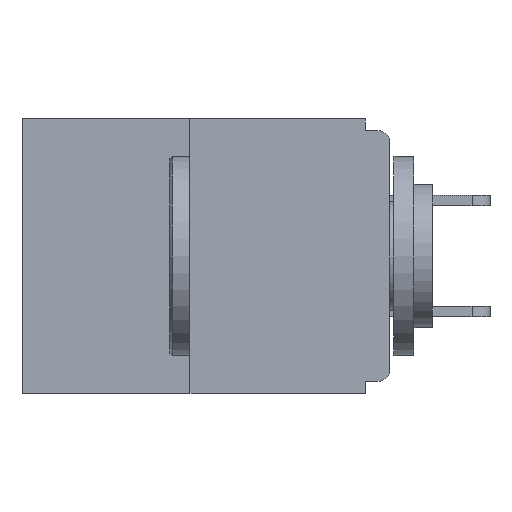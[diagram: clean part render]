
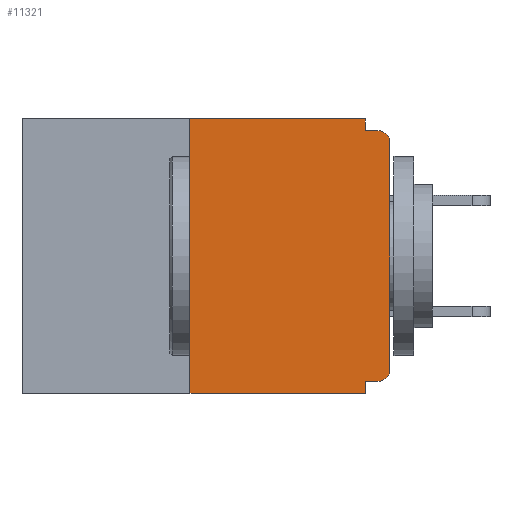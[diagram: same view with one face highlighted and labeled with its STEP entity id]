
A CAD part, left-side view. The second image highlights one B-rep face of the part: STEP entity #11321.
In plain terms, the highlighted planar face has unit normal (-1, 0, 0).
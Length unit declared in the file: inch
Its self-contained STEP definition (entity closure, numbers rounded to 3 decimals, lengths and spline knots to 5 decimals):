
#29 = DIRECTION ( 'NONE',  ( 1., 0., 0. ) ) ;
#92 = ORIENTED_EDGE ( 'NONE', *, *, #10430, .T. ) ;
#183 = DIRECTION ( 'NONE',  ( 0., 0., 1. ) ) ;
#294 = VERTEX_POINT ( 'NONE', #725 ) ;
#322 = AXIS2_PLACEMENT_3D ( 'NONE', #8437, #29, #8580 ) ;
#725 = CARTESIAN_POINT ( 'NONE',  ( 0., 0., -0.313 ) ) ;
#893 = CARTESIAN_POINT ( 'NONE',  ( 0., 0.031, -0.343 ) ) ;
#1575 = CARTESIAN_POINT ( 'NONE',  ( 0., 0.25, 0. ) ) ;
#1638 = DIRECTION ( 'NONE',  ( 0., 0., -1. ) ) ;
#2062 = ORIENTED_EDGE ( 'NONE', *, *, #11120, .T. ) ;
#2127 = LINE ( 'NONE', #3021, #7618 ) ;
#2630 = DIRECTION ( 'NONE',  ( 0., 0., -1. ) ) ;
#3021 = CARTESIAN_POINT ( 'NONE',  ( 0., 0.46, -0.343 ) ) ;
#3140 = CARTESIAN_POINT ( 'NONE',  ( 0., 0.031, -0.015 ) ) ;
#3347 = ORIENTED_EDGE ( 'NONE', *, *, #10351, .T. ) ;
#3365 = ORIENTED_EDGE ( 'NONE', *, *, #12907, .F. ) ;
#3412 = LINE ( 'NONE', #9263, #6564 ) ;
#3516 = CARTESIAN_POINT ( 'NONE',  ( 0., 0.015, -0.03 ) ) ;
#3700 = EDGE_CURVE ( 'NONE', #9054, #10824, #12797, .T. ) ;
#4074 = DIRECTION ( 'NONE',  ( 0., -1., 0. ) ) ;
#4502 = VECTOR ( 'NONE', #12166, 39.37008 ) ;
#4581 = CARTESIAN_POINT ( 'NONE',  ( 0., 0.25, 0. ) ) ;
#4733 = VECTOR ( 'NONE', #7229, 39.37008 ) ;
#4738 = DIRECTION ( 'NONE',  ( -1., 0., 0. ) ) ;
#4874 = EDGE_CURVE ( 'NONE', #5686, #12317, #10816, .T. ) ;
#5145 = CARTESIAN_POINT ( 'NONE',  ( 0., 0.46, 0. ) ) ;
#5292 = CARTESIAN_POINT ( 'NONE',  ( 0., 0.015, -0.328 ) ) ;
#5483 = VECTOR ( 'NONE', #4074, 39.37008 ) ;
#5686 = VERTEX_POINT ( 'NONE', #3140 ) ;
#5849 = ORIENTED_EDGE ( 'NONE', *, *, #12723, .F. ) ;
#5891 = DIRECTION ( 'NONE',  ( 0., 0., 1. ) ) ;
#6254 = LINE ( 'NONE', #4581, #9933 ) ;
#6564 = VECTOR ( 'NONE', #12389, 39.37008 ) ;
#7229 = DIRECTION ( 'NONE',  ( 0., -1., 0. ) ) ;
#7510 = VERTEX_POINT ( 'NONE', #8143 ) ;
#7606 = CIRCLE ( 'NONE', #13132, 0.015 ) ;
#7618 = VECTOR ( 'NONE', #11490, 39.37008 ) ;
#7739 = VECTOR ( 'NONE', #1638, 39.37008 ) ;
#7853 = ORIENTED_EDGE ( 'NONE', *, *, #4874, .F. ) ;
#7925 = VERTEX_POINT ( 'NONE', #893 ) ;
#8143 = CARTESIAN_POINT ( 'NONE',  ( 0., 0.25, -0.343 ) ) ;
#8423 = DIRECTION ( 'NONE',  ( 0., 0., -1. ) ) ;
#8437 = CARTESIAN_POINT ( 'NONE',  ( 0., 0.46, 0. ) ) ;
#8442 = ORIENTED_EDGE ( 'NONE', *, *, #3700, .F. ) ;
#8482 = PLANE ( 'NONE',  #322 ) ;
#8580 = DIRECTION ( 'NONE',  ( 0., 0., -1. ) ) ;
#9054 = VERTEX_POINT ( 'NONE', #5292 ) ;
#9079 = CARTESIAN_POINT ( 'NONE',  ( 0., 0.031, -0.328 ) ) ;
#9081 = ORIENTED_EDGE ( 'NONE', *, *, #13588, .F. ) ;
#9259 = CARTESIAN_POINT ( 'NONE',  ( 0., 0., -0.015 ) ) ;
#9263 = CARTESIAN_POINT ( 'NONE',  ( 0., 0.031, -0.343 ) ) ;
#9368 = CARTESIAN_POINT ( 'NONE',  ( 0., 0.015, -0.313 ) ) ;
#9779 = CARTESIAN_POINT ( 'NONE',  ( 0., 0.015, -0.015 ) ) ;
#9899 = LINE ( 'NONE', #5145, #4733 ) ;
#9933 = VECTOR ( 'NONE', #5891, 39.37008 ) ;
#10029 = CARTESIAN_POINT ( 'NONE',  ( 0., 0., -0.03 ) ) ;
#10239 = ORIENTED_EDGE ( 'NONE', *, *, #13174, .T. ) ;
#10351 = EDGE_CURVE ( 'NONE', #9054, #294, #11297, .T. ) ;
#10430 = EDGE_CURVE ( 'NONE', #7510, #7925, #2127, .T. ) ;
#10437 = FACE_OUTER_BOUND ( 'NONE', #10765, .T. ) ;
#10654 = CARTESIAN_POINT ( 'NONE',  ( 0., 0., 0. ) ) ;
#10765 = EDGE_LOOP ( 'NONE', ( #9081, #5849, #92, #3365, #8442, #3347, #10239, #2062, #7853, #12863 ) ) ;
#10806 = VERTEX_POINT ( 'NONE', #10029 ) ;
#10816 = LINE ( 'NONE', #9259, #5483 ) ;
#10824 = VERTEX_POINT ( 'NONE', #9079 ) ;
#11067 = VECTOR ( 'NONE', #183, 39.37008 ) ;
#11120 = EDGE_CURVE ( 'NONE', #10806, #12317, #7606, .T. ) ;
#11126 = CARTESIAN_POINT ( 'NONE',  ( 0., 0.031, 0. ) ) ;
#11297 = CIRCLE ( 'NONE', #11362, 0.015 ) ;
#11321 = ADVANCED_FACE ( 'NONE', ( #10437 ), #8482, .F. ) ;
#11362 = AXIS2_PLACEMENT_3D ( 'NONE', #9368, #13664, #8423 ) ;
#11453 = CARTESIAN_POINT ( 'NONE',  ( 0., 0.031, 0. ) ) ;
#11490 = DIRECTION ( 'NONE',  ( 0., -1., 0. ) ) ;
#12076 = CARTESIAN_POINT ( 'NONE',  ( 0., 0., -0.328 ) ) ;
#12166 = DIRECTION ( 'NONE',  ( 0., 1., 0. ) ) ;
#12317 = VERTEX_POINT ( 'NONE', #9779 ) ;
#12389 = DIRECTION ( 'NONE',  ( 0., 0., -1. ) ) ;
#12494 = EDGE_CURVE ( 'NONE', #13684, #5686, #13400, .T. ) ;
#12723 = EDGE_CURVE ( 'NONE', #7510, #13493, #6254, .T. ) ;
#12797 = LINE ( 'NONE', #12076, #4502 ) ;
#12863 = ORIENTED_EDGE ( 'NONE', *, *, #12494, .F. ) ;
#12907 = EDGE_CURVE ( 'NONE', #10824, #7925, #3412, .T. ) ;
#13132 = AXIS2_PLACEMENT_3D ( 'NONE', #3516, #4738, #2630 ) ;
#13174 = EDGE_CURVE ( 'NONE', #294, #10806, #13373, .T. ) ;
#13373 = LINE ( 'NONE', #10654, #11067 ) ;
#13400 = LINE ( 'NONE', #11126, #7739 ) ;
#13493 = VERTEX_POINT ( 'NONE', #1575 ) ;
#13588 = EDGE_CURVE ( 'NONE', #13493, #13684, #9899, .T. ) ;
#13664 = DIRECTION ( 'NONE',  ( -1., 0., 0. ) ) ;
#13684 = VERTEX_POINT ( 'NONE', #11453 ) ;
